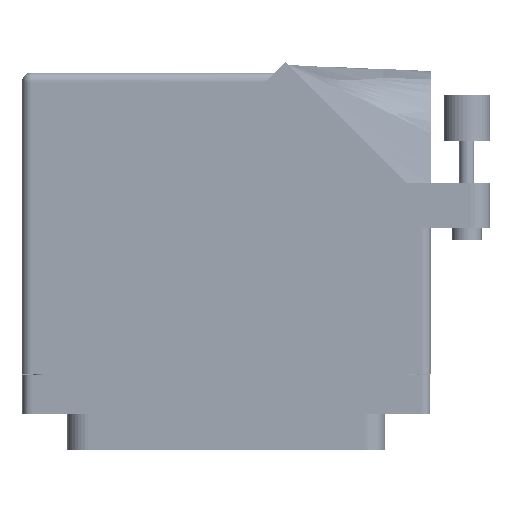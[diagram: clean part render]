
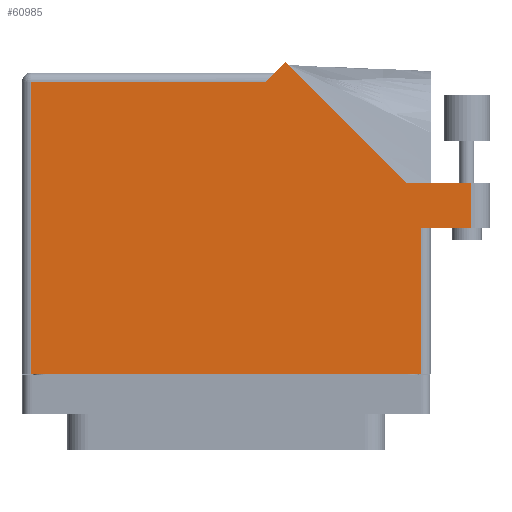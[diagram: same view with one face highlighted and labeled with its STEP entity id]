
A CAD part, front view. The second image highlights one B-rep face of the part: STEP entity #60985.
In plain terms, the highlighted face is planar.
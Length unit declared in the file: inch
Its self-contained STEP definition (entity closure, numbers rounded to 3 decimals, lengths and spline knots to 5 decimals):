
#671 = VERTEX_POINT ( 'NONE', #37113 ) ;
#1112 = CARTESIAN_POINT ( 'NONE',  ( 1.3155, -0.1, 0.765 ) ) ;
#1810 = EDGE_CURVE ( 'NONE', #47708, #4070, #38615, .T. ) ;
#2571 = CARTESIAN_POINT ( 'NONE',  ( 0.39821, 2.00071, 0.765 ) ) ;
#4070 = VERTEX_POINT ( 'NONE', #40641 ) ;
#4226 = PLANE ( 'NONE',  #55197 ) ;
#4342 = EDGE_CURVE ( 'NONE', #4070, #4603, #12198, .T. ) ;
#4603 = VERTEX_POINT ( 'NONE', #21595 ) ;
#5150 = DIRECTION ( 'NONE',  ( 0., 1., 0. ) ) ;
#8042 = VERTEX_POINT ( 'NONE', #2571 ) ;
#9999 = VECTOR ( 'NONE', #5150, 39.37008 ) ;
#10378 = EDGE_CURVE ( 'NONE', #39746, #47708, #22356, .T. ) ;
#10489 = DIRECTION ( 'NONE',  ( 0., -1., 0. ) ) ;
#10808 = CARTESIAN_POINT ( 'NONE',  ( -1.3155, -0.1, 0.765 ) ) ;
#11176 = DIRECTION ( 'NONE',  ( 0., 0., -1. ) ) ;
#12198 = LINE ( 'NONE', #24889, #9999 ) ;
#13192 = DIRECTION ( 'NONE',  ( -1., 0., 0. ) ) ;
#14873 = LINE ( 'NONE', #76807, #17007 ) ;
#15300 = ORIENTED_EDGE ( 'NONE', *, *, #75592, .T. ) ;
#16048 = CARTESIAN_POINT ( 'NONE',  ( 1.3155, 0.88, 0.765 ) ) ;
#17007 = VECTOR ( 'NONE', #35501, 39.37008 ) ;
#17213 = VECTOR ( 'NONE', #13192, 39.37008 ) ;
#17574 = CARTESIAN_POINT ( 'NONE',  ( 1.21192, 1.187, 0.765 ) ) ;
#17863 = DIRECTION ( 'NONE',  ( -1., 0., 0. ) ) ;
#18134 = CARTESIAN_POINT ( 'NONE',  ( -1.3775, 1.93, 0.765 ) ) ;
#18842 = DIRECTION ( 'NONE',  ( -0.707, -0.707, 0. ) ) ;
#20438 = VERTEX_POINT ( 'NONE', #80838 ) ;
#21188 = CARTESIAN_POINT ( 'NONE',  ( 1.3155, 0.88, 0.765 ) ) ;
#21595 = CARTESIAN_POINT ( 'NONE',  ( 1.6525, 1.187, 0.765 ) ) ;
#22068 = ORIENTED_EDGE ( 'NONE', *, *, #40845, .T. ) ;
#22356 = LINE ( 'NONE', #21188, #55811 ) ;
#23374 = ORIENTED_EDGE ( 'NONE', *, *, #54058, .T. ) ;
#24865 = ORIENTED_EDGE ( 'NONE', *, *, #4342, .T. ) ;
#24889 = CARTESIAN_POINT ( 'NONE',  ( 1.6525, 1.187, 0.765 ) ) ;
#25661 = VECTOR ( 'NONE', #10489, 39.37008 ) ;
#28216 = ORIENTED_EDGE ( 'NONE', *, *, #55816, .T. ) ;
#32335 = ORIENTED_EDGE ( 'NONE', *, *, #39377, .T. ) ;
#34208 = LINE ( 'NONE', #17574, #59040 ) ;
#35501 = DIRECTION ( 'NONE',  ( 1., 0., 0. ) ) ;
#36034 = ORIENTED_EDGE ( 'NONE', *, *, #1810, .T. ) ;
#37113 = CARTESIAN_POINT ( 'NONE',  ( -1.3155, -0.1, 0.765 ) ) ;
#38414 = VERTEX_POINT ( 'NONE', #70609 ) ;
#38615 = LINE ( 'NONE', #86630, #82782 ) ;
#39377 = EDGE_CURVE ( 'NONE', #38414, #671, #83858, .T. ) ;
#39746 = VERTEX_POINT ( 'NONE', #1112 ) ;
#40641 = CARTESIAN_POINT ( 'NONE',  ( 1.6525, 0.88, 0.765 ) ) ;
#40845 = EDGE_CURVE ( 'NONE', #671, #39746, #14873, .T. ) ;
#44791 = EDGE_CURVE ( 'NONE', #20438, #8042, #34208, .T. ) ;
#45966 = VECTOR ( 'NONE', #73050, 39.37008 ) ;
#46193 = DIRECTION ( 'NONE',  ( 1., 0., 0. ) ) ;
#47708 = VERTEX_POINT ( 'NONE', #16048 ) ;
#48628 = CARTESIAN_POINT ( 'NONE',  ( 0.2655, 1.868, 0.765 ) ) ;
#53511 = CARTESIAN_POINT ( 'NONE',  ( 0.3275, 1.93, 0.765 ) ) ;
#54058 = EDGE_CURVE ( 'NONE', #4603, #20438, #86277, .T. ) ;
#55197 = AXIS2_PLACEMENT_3D ( 'NONE', #18134, #11176, #17863 ) ;
#55811 = VECTOR ( 'NONE', #83014, 39.37008 ) ;
#55816 = EDGE_CURVE ( 'NONE', #67150, #38414, #76147, .T. ) ;
#57795 = LINE ( 'NONE', #53511, #85846 ) ;
#59040 = VECTOR ( 'NONE', #66180, 39.37008 ) ;
#60985 = ADVANCED_FACE ( 'NONE', ( #79257 ), #4226, .F. ) ;
#62060 = CARTESIAN_POINT ( 'NONE',  ( 1.7775, 1.187, 0.765 ) ) ;
#63460 = ORIENTED_EDGE ( 'NONE', *, *, #10378, .T. ) ;
#63894 = ORIENTED_EDGE ( 'NONE', *, *, #44791, .T. ) ;
#66180 = DIRECTION ( 'NONE',  ( -0.707, 0.707, 0. ) ) ;
#67150 = VERTEX_POINT ( 'NONE', #48628 ) ;
#70609 = CARTESIAN_POINT ( 'NONE',  ( -1.3155, 1.868, 0.765 ) ) ;
#73050 = DIRECTION ( 'NONE',  ( -1., 0., 0. ) ) ;
#75592 = EDGE_CURVE ( 'NONE', #8042, #67150, #57795, .T. ) ;
#76147 = LINE ( 'NONE', #86905, #45966 ) ;
#76807 = CARTESIAN_POINT ( 'NONE',  ( -1.3775, -0.1, 0.765 ) ) ;
#79102 = EDGE_LOOP ( 'NONE', ( #36034, #24865, #23374, #63894, #15300, #28216, #32335, #22068, #63460 ) ) ;
#79257 = FACE_OUTER_BOUND ( 'NONE', #79102, .T. ) ;
#80838 = CARTESIAN_POINT ( 'NONE',  ( 1.21192, 1.187, 0.765 ) ) ;
#82782 = VECTOR ( 'NONE', #46193, 39.37008 ) ;
#83014 = DIRECTION ( 'NONE',  ( 0., 1., 0. ) ) ;
#83858 = LINE ( 'NONE', #10808, #25661 ) ;
#85846 = VECTOR ( 'NONE', #18842, 39.37008 ) ;
#86277 = LINE ( 'NONE', #62060, #17213 ) ;
#86630 = CARTESIAN_POINT ( 'NONE',  ( 1.3775, 0.88, 0.765 ) ) ;
#86905 = CARTESIAN_POINT ( 'NONE',  ( -1.3775, 1.868, 0.765 ) ) ;
